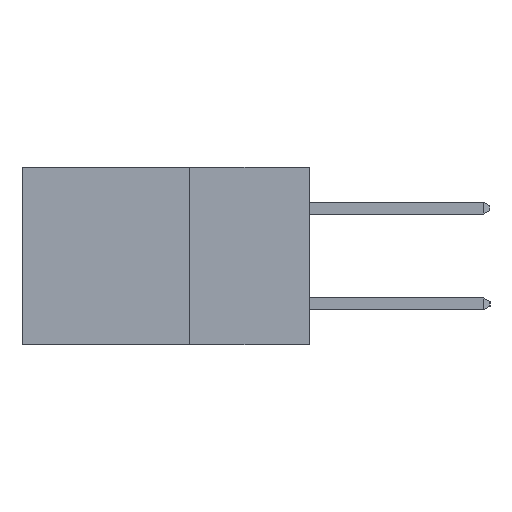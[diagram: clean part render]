
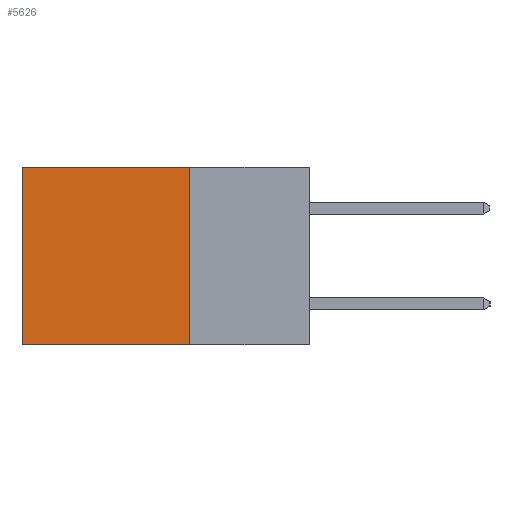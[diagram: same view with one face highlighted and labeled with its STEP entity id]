
A CAD part, left-side view. The second image highlights one B-rep face of the part: STEP entity #5626.
In plain terms, the highlighted planar face has unit normal (-1, 0, 0).
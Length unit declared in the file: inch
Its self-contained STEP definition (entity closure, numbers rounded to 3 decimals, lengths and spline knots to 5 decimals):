
#399 = LINE ( 'NONE', #12153, #9744 ) ;
#538 = CARTESIAN_POINT ( 'NONE',  ( 0.2875, 0.25, -0.37 ) ) ;
#642 = DIRECTION ( 'NONE',  ( 0., 1., 0. ) ) ;
#756 = PLANE ( 'NONE',  #10774 ) ;
#967 = EDGE_LOOP ( 'NONE', ( #7677, #1823, #12774, #5303 ) ) ;
#1388 = LINE ( 'NONE', #8281, #2060 ) ;
#1823 = ORIENTED_EDGE ( 'NONE', *, *, #7923, .F. ) ;
#2060 = VECTOR ( 'NONE', #3050, 39.37008 ) ;
#2257 = CARTESIAN_POINT ( 'NONE',  ( 0.2875, 0.6, -0.37 ) ) ;
#3050 = DIRECTION ( 'NONE',  ( 0., 0., -1. ) ) ;
#3109 = EDGE_CURVE ( 'NONE', #3310, #11846, #1388, .T. ) ;
#3310 = VERTEX_POINT ( 'NONE', #7517 ) ;
#3763 = DIRECTION ( 'NONE',  ( 0., 0., -1. ) ) ;
#3932 = VERTEX_POINT ( 'NONE', #4488 ) ;
#4151 = EDGE_CURVE ( 'NONE', #3932, #3310, #399, .T. ) ;
#4488 = CARTESIAN_POINT ( 'NONE',  ( 0.2875, 0.25, 0. ) ) ;
#5303 = ORIENTED_EDGE ( 'NONE', *, *, #4151, .T. ) ;
#5521 = FACE_OUTER_BOUND ( 'NONE', #967, .T. ) ;
#5626 = ADVANCED_FACE ( 'NONE', ( #5521 ), #756, .F. ) ;
#5881 = VERTEX_POINT ( 'NONE', #538 ) ;
#6010 = EDGE_CURVE ( 'NONE', #3932, #5881, #10314, .T. ) ;
#6497 = VECTOR ( 'NONE', #3763, 39.37008 ) ;
#7517 = CARTESIAN_POINT ( 'NONE',  ( 0.2875, 0.6, 0. ) ) ;
#7677 = ORIENTED_EDGE ( 'NONE', *, *, #3109, .T. ) ;
#7923 = EDGE_CURVE ( 'NONE', #5881, #11846, #13019, .T. ) ;
#8281 = CARTESIAN_POINT ( 'NONE',  ( 0.2875, 0.6, 0. ) ) ;
#9067 = CARTESIAN_POINT ( 'NONE',  ( 0.2875, 0.25, 0. ) ) ;
#9188 = CARTESIAN_POINT ( 'NONE',  ( 0.2875, 0.25, 0. ) ) ;
#9384 = CARTESIAN_POINT ( 'NONE',  ( 0.2875, 0.25, -0.37 ) ) ;
#9617 = VECTOR ( 'NONE', #12111, 39.37008 ) ;
#9744 = VECTOR ( 'NONE', #642, 39.37008 ) ;
#10314 = LINE ( 'NONE', #9067, #6497 ) ;
#10774 = AXIS2_PLACEMENT_3D ( 'NONE', #9188, #13324, #11435 ) ;
#11435 = DIRECTION ( 'NONE',  ( 0., 0., -1. ) ) ;
#11846 = VERTEX_POINT ( 'NONE', #2257 ) ;
#12111 = DIRECTION ( 'NONE',  ( 0., 1., 0. ) ) ;
#12153 = CARTESIAN_POINT ( 'NONE',  ( 0.2875, 0.25, 0. ) ) ;
#12774 = ORIENTED_EDGE ( 'NONE', *, *, #6010, .F. ) ;
#13019 = LINE ( 'NONE', #9384, #9617 ) ;
#13324 = DIRECTION ( 'NONE',  ( 1., 0., 0. ) ) ;
